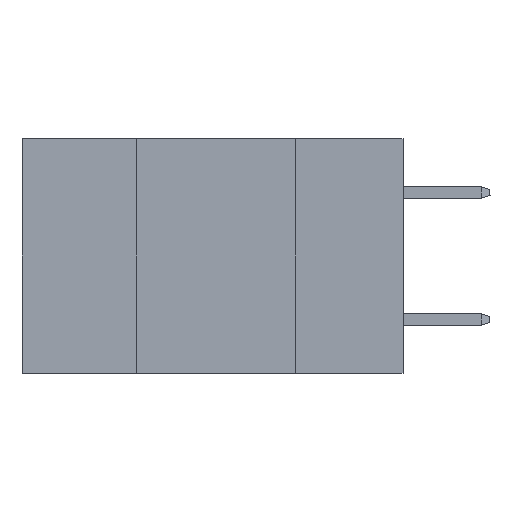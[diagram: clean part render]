
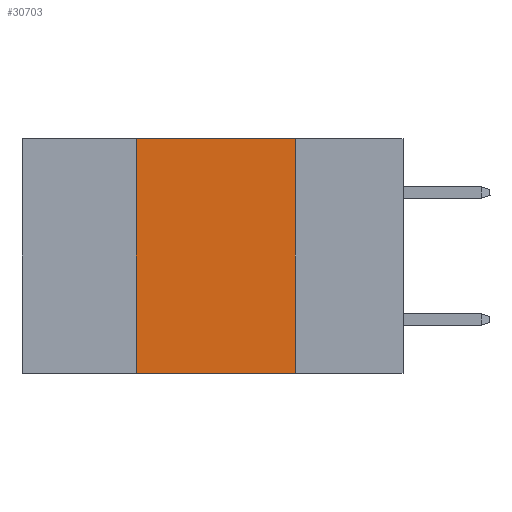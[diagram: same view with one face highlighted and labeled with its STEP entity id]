
A CAD part, left-side view. The second image highlights one B-rep face of the part: STEP entity #30703.
In plain terms, the highlighted planar face has unit normal (-1, 0, 0).
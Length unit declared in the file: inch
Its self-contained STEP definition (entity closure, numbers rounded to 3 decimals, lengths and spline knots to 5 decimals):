
#1341 = AXIS2_PLACEMENT_3D ( 'NONE', #12051, #3566, #6705 ) ;
#1344 = LINE ( 'NONE', #35091, #15733 ) ;
#2221 = EDGE_CURVE ( 'NONE', #10050, #20631, #33580, .T. ) ;
#3435 = DIRECTION ( 'NONE',  ( 0., -1., 0. ) ) ;
#3566 = DIRECTION ( 'NONE',  ( 1., 0., 0. ) ) ;
#4724 = EDGE_CURVE ( 'NONE', #18651, #5375, #30339, .T. ) ;
#5375 = VERTEX_POINT ( 'NONE', #19400 ) ;
#6325 = EDGE_LOOP ( 'NONE', ( #34253, #21645, #17215, #8609 ) ) ;
#6705 = DIRECTION ( 'NONE',  ( 0., 0., -1. ) ) ;
#6713 = DIRECTION ( 'NONE',  ( 0., -1., 0. ) ) ;
#7548 = VECTOR ( 'NONE', #22335, 39.37008 ) ;
#8609 = ORIENTED_EDGE ( 'NONE', *, *, #31481, .T. ) ;
#9465 = FACE_OUTER_BOUND ( 'NONE', #6325, .T. ) ;
#10050 = VERTEX_POINT ( 'NONE', #23304 ) ;
#12051 = CARTESIAN_POINT ( 'NONE',  ( 0., 0.6, 0. ) ) ;
#13550 = CARTESIAN_POINT ( 'NONE',  ( 0., 0.42, 0. ) ) ;
#15733 = VECTOR ( 'NONE', #6713, 39.37008 ) ;
#17215 = ORIENTED_EDGE ( 'NONE', *, *, #4724, .F. ) ;
#17783 = CARTESIAN_POINT ( 'NONE',  ( 0., 0.42, -0.37 ) ) ;
#17812 = LINE ( 'NONE', #32011, #18384 ) ;
#18384 = VECTOR ( 'NONE', #3435, 39.37008 ) ;
#18651 = VERTEX_POINT ( 'NONE', #17783 ) ;
#19400 = CARTESIAN_POINT ( 'NONE',  ( 0., 0.42, 0. ) ) ;
#20631 = VERTEX_POINT ( 'NONE', #28470 ) ;
#21645 = ORIENTED_EDGE ( 'NONE', *, *, #22164, .F. ) ;
#22164 = EDGE_CURVE ( 'NONE', #5375, #10050, #1344, .T. ) ;
#22335 = DIRECTION ( 'NONE',  ( 0., 0., -1. ) ) ;
#22947 = PLANE ( 'NONE',  #1341 ) ;
#23304 = CARTESIAN_POINT ( 'NONE',  ( 0., 0.17, 0. ) ) ;
#24432 = VECTOR ( 'NONE', #24801, 39.37008 ) ;
#24801 = DIRECTION ( 'NONE',  ( 0., 0., 1. ) ) ;
#27863 = CARTESIAN_POINT ( 'NONE',  ( 0., 0.17, 0. ) ) ;
#28470 = CARTESIAN_POINT ( 'NONE',  ( 0., 0.17, -0.37 ) ) ;
#30339 = LINE ( 'NONE', #13550, #24432 ) ;
#30703 = ADVANCED_FACE ( 'NONE', ( #9465 ), #22947, .F. ) ;
#31481 = EDGE_CURVE ( 'NONE', #18651, #20631, #17812, .T. ) ;
#32011 = CARTESIAN_POINT ( 'NONE',  ( 0., 0.6, -0.37 ) ) ;
#33580 = LINE ( 'NONE', #27863, #7548 ) ;
#34253 = ORIENTED_EDGE ( 'NONE', *, *, #2221, .F. ) ;
#35091 = CARTESIAN_POINT ( 'NONE',  ( 0., 0.6, 0. ) ) ;
